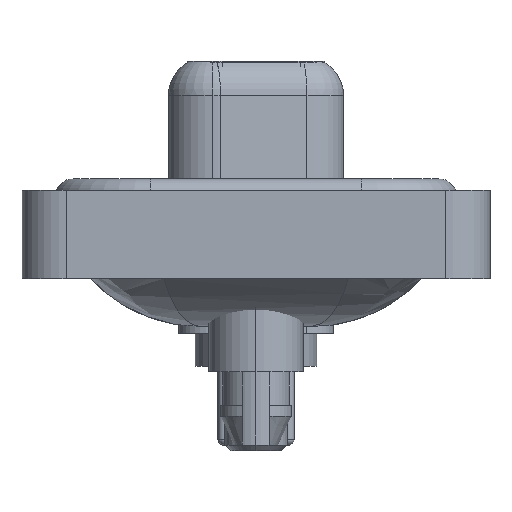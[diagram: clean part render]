
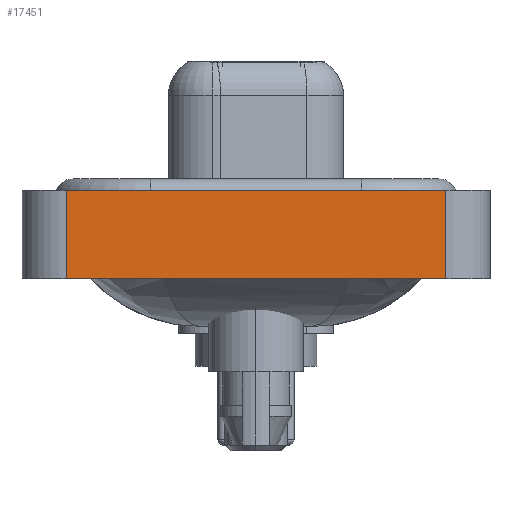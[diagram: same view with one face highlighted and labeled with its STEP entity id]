
A CAD part, left-side view. The second image highlights one B-rep face of the part: STEP entity #17451.
In plain terms, the highlighted planar face has unit normal (-1, 0, 0).
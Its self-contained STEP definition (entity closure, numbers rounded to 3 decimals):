
#213 = VERTEX_POINT ( 'NONE', #19038 ) ;
#836 = DIRECTION ( 'NONE',  ( 0., 0., 1. ) ) ;
#1225 = EDGE_CURVE ( 'NONE', #8018, #12240, #21764, .T. ) ;
#1873 = DIRECTION ( 'NONE',  ( -1., 0., 0. ) ) ;
#2076 = CARTESIAN_POINT ( 'NONE',  ( -7.35, -8.55, 0.4 ) ) ;
#3132 = ORIENTED_EDGE ( 'NONE', *, *, #7120, .F. ) ;
#5586 = LINE ( 'NONE', #11455, #6043 ) ;
#6043 = VECTOR ( 'NONE', #13191, 1000. ) ;
#6484 = DIRECTION ( 'NONE',  ( 0., -1., 0. ) ) ;
#6695 = CARTESIAN_POINT ( 'NONE',  ( -7.35, -8.55, -3.6 ) ) ;
#7120 = EDGE_CURVE ( 'NONE', #213, #16465, #5586, .T. ) ;
#7538 = EDGE_CURVE ( 'NONE', #213, #8018, #15439, .T. ) ;
#8018 = VERTEX_POINT ( 'NONE', #14018 ) ;
#8431 = AXIS2_PLACEMENT_3D ( 'NONE', #11033, #1873, #22642 ) ;
#9820 = ORIENTED_EDGE ( 'NONE', *, *, #7538, .T. ) ;
#9886 = LINE ( 'NONE', #2076, #13908 ) ;
#11033 = CARTESIAN_POINT ( 'NONE',  ( -7.35, -8.55, -3.6 ) ) ;
#11363 = DIRECTION ( 'NONE',  ( 0., -1., 0. ) ) ;
#11455 = CARTESIAN_POINT ( 'NONE',  ( -7.35, 8.55, -3.6 ) ) ;
#12240 = VERTEX_POINT ( 'NONE', #13345 ) ;
#13191 = DIRECTION ( 'NONE',  ( 0., 0., 1. ) ) ;
#13345 = CARTESIAN_POINT ( 'NONE',  ( -7.35, -8.55, 0.4 ) ) ;
#13908 = VECTOR ( 'NONE', #11363, 1000. ) ;
#14018 = CARTESIAN_POINT ( 'NONE',  ( -7.35, -8.55, -3.6 ) ) ;
#14779 = VECTOR ( 'NONE', #836, 1000. ) ;
#15439 = LINE ( 'NONE', #21417, #17014 ) ;
#16465 = VERTEX_POINT ( 'NONE', #22882 ) ;
#16675 = FACE_OUTER_BOUND ( 'NONE', #18543, .T. ) ;
#17014 = VECTOR ( 'NONE', #6484, 1000. ) ;
#17118 = ORIENTED_EDGE ( 'NONE', *, *, #22650, .F. ) ;
#17451 = ADVANCED_FACE ( 'NONE', ( #16675 ), #20817, .T. ) ;
#18543 = EDGE_LOOP ( 'NONE', ( #21726, #17118, #3132, #9820 ) ) ;
#19038 = CARTESIAN_POINT ( 'NONE',  ( -7.35, 8.55, -3.6 ) ) ;
#20817 = PLANE ( 'NONE',  #8431 ) ;
#21417 = CARTESIAN_POINT ( 'NONE',  ( -7.35, -8.55, -3.6 ) ) ;
#21726 = ORIENTED_EDGE ( 'NONE', *, *, #1225, .T. ) ;
#21764 = LINE ( 'NONE', #6695, #14779 ) ;
#22642 = DIRECTION ( 'NONE',  ( 0., 0., 1. ) ) ;
#22650 = EDGE_CURVE ( 'NONE', #16465, #12240, #9886, .T. ) ;
#22882 = CARTESIAN_POINT ( 'NONE',  ( -7.35, 8.55, 0.4 ) ) ;
